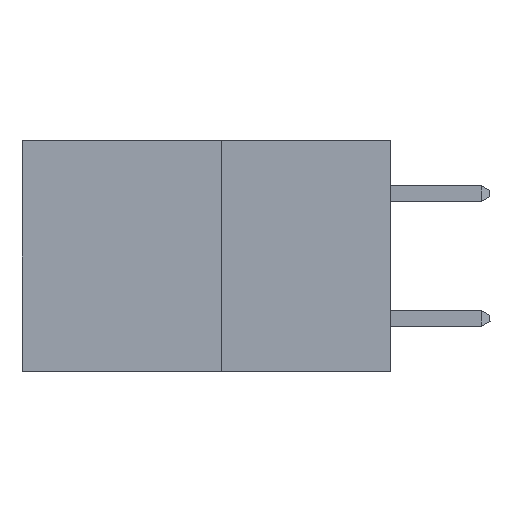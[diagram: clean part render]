
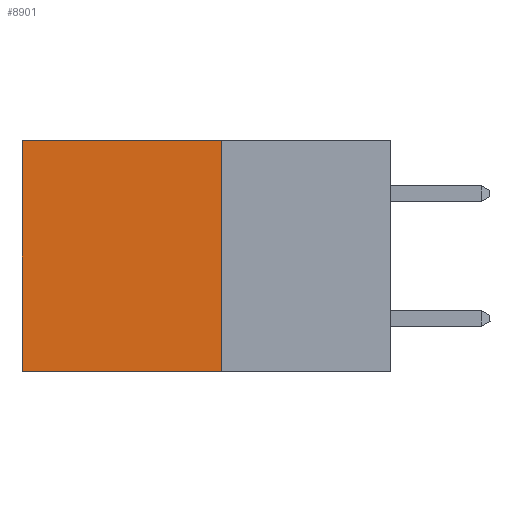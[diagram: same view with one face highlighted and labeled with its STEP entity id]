
A CAD part, left-side view. The second image highlights one B-rep face of the part: STEP entity #8901.
In plain terms, the highlighted planar face has unit normal (-1, 0, 0).
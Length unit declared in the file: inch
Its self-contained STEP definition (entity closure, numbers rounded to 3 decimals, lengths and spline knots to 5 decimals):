
#78 = DIRECTION ( 'NONE',  ( 0., 1., 0. ) ) ;
#1098 = EDGE_LOOP ( 'NONE', ( #5762, #9242, #15155, #13884 ) ) ;
#1136 = CARTESIAN_POINT ( 'NONE',  ( 0.277, 0.59, -0.37 ) ) ;
#1181 = LINE ( 'NONE', #20271, #16273 ) ;
#1253 = AXIS2_PLACEMENT_3D ( 'NONE', #24229, #12854, #1526 ) ;
#1526 = DIRECTION ( 'NONE',  ( 0., 0., -1. ) ) ;
#1818 = EDGE_CURVE ( 'NONE', #4292, #16057, #8313, .T. ) ;
#1929 = VECTOR ( 'NONE', #16266, 39.37008 ) ;
#4292 = VERTEX_POINT ( 'NONE', #13044 ) ;
#5757 = CARTESIAN_POINT ( 'NONE',  ( 0.277, 0.27, 0. ) ) ;
#5762 = ORIENTED_EDGE ( 'NONE', *, *, #23893, .T. ) ;
#6230 = EDGE_CURVE ( 'NONE', #4292, #12310, #20267, .T. ) ;
#7718 = VECTOR ( 'NONE', #21887, 39.37008 ) ;
#8313 = LINE ( 'NONE', #8577, #7718 ) ;
#8577 = CARTESIAN_POINT ( 'NONE',  ( 0.277, 0.27, -0.37 ) ) ;
#8812 = EDGE_CURVE ( 'NONE', #16057, #18702, #1181, .T. ) ;
#8858 = DIRECTION ( 'NONE',  ( 0., 1., 0. ) ) ;
#8901 = ADVANCED_FACE ( 'NONE', ( #23989 ), #10909, .F. ) ;
#9242 = ORIENTED_EDGE ( 'NONE', *, *, #8812, .F. ) ;
#9360 = CARTESIAN_POINT ( 'NONE',  ( 0.277, 0.27, -0.37 ) ) ;
#10122 = VECTOR ( 'NONE', #78, 39.37008 ) ;
#10909 = PLANE ( 'NONE',  #1253 ) ;
#12310 = VERTEX_POINT ( 'NONE', #17445 ) ;
#12854 = DIRECTION ( 'NONE',  ( 1., 0., 0. ) ) ;
#13044 = CARTESIAN_POINT ( 'NONE',  ( 0.277, 0.27, 0. ) ) ;
#13884 = ORIENTED_EDGE ( 'NONE', *, *, #6230, .T. ) ;
#15155 = ORIENTED_EDGE ( 'NONE', *, *, #1818, .F. ) ;
#16057 = VERTEX_POINT ( 'NONE', #9360 ) ;
#16266 = DIRECTION ( 'NONE',  ( 0., 0., -1. ) ) ;
#16273 = VECTOR ( 'NONE', #8858, 39.37008 ) ;
#17445 = CARTESIAN_POINT ( 'NONE',  ( 0.277, 0.59, 0. ) ) ;
#18702 = VERTEX_POINT ( 'NONE', #23608 ) ;
#20267 = LINE ( 'NONE', #5757, #10122 ) ;
#20271 = CARTESIAN_POINT ( 'NONE',  ( 0.277, 0.27, -0.37 ) ) ;
#21887 = DIRECTION ( 'NONE',  ( 0., 0., -1. ) ) ;
#22116 = LINE ( 'NONE', #1136, #1929 ) ;
#23608 = CARTESIAN_POINT ( 'NONE',  ( 0.277, 0.59, -0.37 ) ) ;
#23893 = EDGE_CURVE ( 'NONE', #12310, #18702, #22116, .T. ) ;
#23989 = FACE_OUTER_BOUND ( 'NONE', #1098, .T. ) ;
#24229 = CARTESIAN_POINT ( 'NONE',  ( 0.277, 0.27, -0.37 ) ) ;
